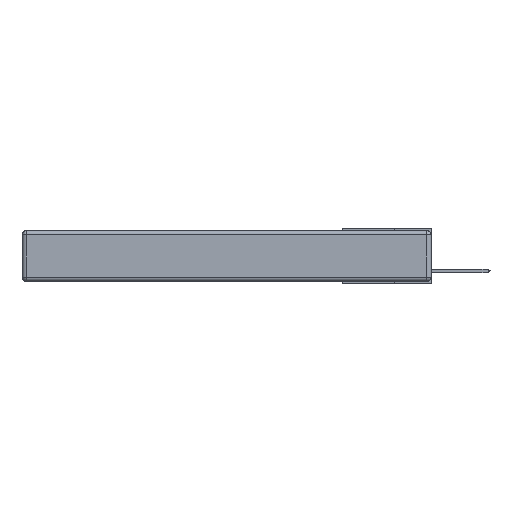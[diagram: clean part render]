
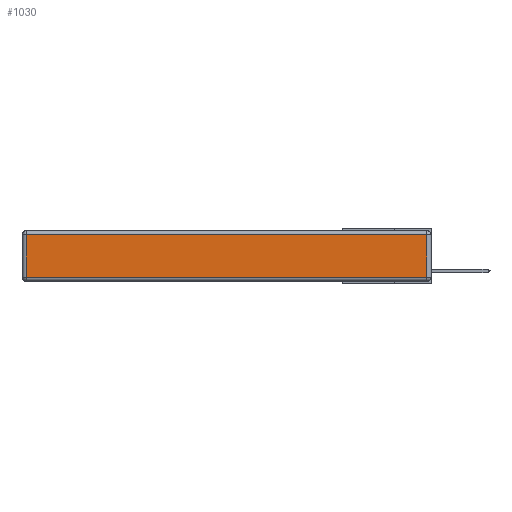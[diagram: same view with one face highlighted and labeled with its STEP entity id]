
A CAD part, left-side view. The second image highlights one B-rep face of the part: STEP entity #1030.
In plain terms, the highlighted planar face has unit normal (-1, 0, 0).
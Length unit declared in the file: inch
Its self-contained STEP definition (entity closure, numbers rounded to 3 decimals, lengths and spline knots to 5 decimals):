
#378 = VERTEX_POINT ( 'NONE', #13031 ) ;
#1030 = ADVANCED_FACE ( 'NONE', ( #24988 ), #20220, .T. ) ;
#1040 = ORIENTED_EDGE ( 'NONE', *, *, #25350, .T. ) ;
#1167 = CARTESIAN_POINT ( 'NONE',  ( 0., 0., -0.313 ) ) ;
#1461 = LINE ( 'NONE', #6703, #25100 ) ;
#3237 = VECTOR ( 'NONE', #6911, 39.37008 ) ;
#3506 = CARTESIAN_POINT ( 'NONE',  ( 0., 2.72, -0.313 ) ) ;
#5758 = LINE ( 'NONE', #11786, #14696 ) ;
#6703 = CARTESIAN_POINT ( 'NONE',  ( 0., 2.72, -0.343 ) ) ;
#6911 = DIRECTION ( 'NONE',  ( 0., -1., 0. ) ) ;
#7058 = EDGE_CURVE ( 'NONE', #18552, #18503, #17069, .T. ) ;
#8414 = DIRECTION ( 'NONE',  ( -1., 0., 0. ) ) ;
#8773 = ORIENTED_EDGE ( 'NONE', *, *, #10781, .T. ) ;
#9526 = CARTESIAN_POINT ( 'NONE',  ( 0., 2.75, -0.03 ) ) ;
#10362 = EDGE_LOOP ( 'NONE', ( #24431, #1040, #8773, #11917 ) ) ;
#10662 = VERTEX_POINT ( 'NONE', #20082 ) ;
#10781 = EDGE_CURVE ( 'NONE', #10662, #378, #24541, .T. ) ;
#11786 = CARTESIAN_POINT ( 'NONE',  ( 0., 0.03, -0.343 ) ) ;
#11917 = ORIENTED_EDGE ( 'NONE', *, *, #15770, .T. ) ;
#13031 = CARTESIAN_POINT ( 'NONE',  ( 0., 2.72, -0.03 ) ) ;
#14137 = VECTOR ( 'NONE', #15577, 39.37008 ) ;
#14696 = VECTOR ( 'NONE', #17677, 39.37008 ) ;
#15577 = DIRECTION ( 'NONE',  ( 0., 1., 0. ) ) ;
#15770 = EDGE_CURVE ( 'NONE', #378, #18552, #1461, .T. ) ;
#16093 = DIRECTION ( 'NONE',  ( 0., 0., 1. ) ) ;
#17069 = LINE ( 'NONE', #1167, #3237 ) ;
#17677 = DIRECTION ( 'NONE',  ( 0., 0., 1. ) ) ;
#18237 = CARTESIAN_POINT ( 'NONE',  ( 0., 0., -0.343 ) ) ;
#18503 = VERTEX_POINT ( 'NONE', #24085 ) ;
#18552 = VERTEX_POINT ( 'NONE', #3506 ) ;
#20004 = AXIS2_PLACEMENT_3D ( 'NONE', #18237, #8414, #16093 ) ;
#20082 = CARTESIAN_POINT ( 'NONE',  ( 0., 0.03, -0.03 ) ) ;
#20220 = PLANE ( 'NONE',  #20004 ) ;
#22520 = DIRECTION ( 'NONE',  ( 0., 0., -1. ) ) ;
#24085 = CARTESIAN_POINT ( 'NONE',  ( 0., 0.03, -0.313 ) ) ;
#24431 = ORIENTED_EDGE ( 'NONE', *, *, #7058, .T. ) ;
#24541 = LINE ( 'NONE', #9526, #14137 ) ;
#24988 = FACE_OUTER_BOUND ( 'NONE', #10362, .T. ) ;
#25100 = VECTOR ( 'NONE', #22520, 39.37008 ) ;
#25350 = EDGE_CURVE ( 'NONE', #18503, #10662, #5758, .T. ) ;
